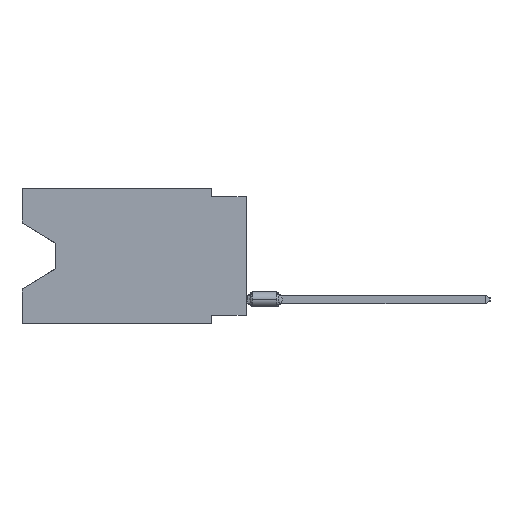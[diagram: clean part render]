
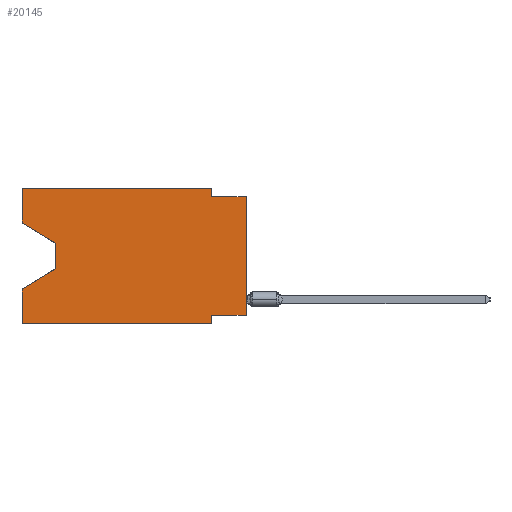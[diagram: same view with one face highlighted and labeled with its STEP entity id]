
A CAD part, left-side view. The second image highlights one B-rep face of the part: STEP entity #20145.
In plain terms, the highlighted planar face has unit normal (-1, 0, 0).
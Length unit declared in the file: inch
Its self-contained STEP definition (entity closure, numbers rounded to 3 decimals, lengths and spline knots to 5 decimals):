
#179 = VERTEX_POINT ( 'NONE', #20235 ) ;
#3113 = VERTEX_POINT ( 'NONE', #60372 ) ;
#4056 = ORIENTED_EDGE ( 'NONE', *, *, #14841, .F. ) ;
#4357 = ORIENTED_EDGE ( 'NONE', *, *, #53268, .F. ) ;
#5197 = EDGE_CURVE ( 'NONE', #50415, #5740, #31365, .T. ) ;
#5271 = ORIENTED_EDGE ( 'NONE', *, *, #59676, .F. ) ;
#5649 = CARTESIAN_POINT ( 'NONE',  ( 0., 0.1, 0. ) ) ;
#5740 = VERTEX_POINT ( 'NONE', #42033 ) ;
#7003 = ORIENTED_EDGE ( 'NONE', *, *, #23905, .T. ) ;
#7552 = CARTESIAN_POINT ( 'NONE',  ( 0., 0., -0.025 ) ) ;
#7831 = VERTEX_POINT ( 'NONE', #5649 ) ;
#9618 = ORIENTED_EDGE ( 'NONE', *, *, #47656, .F. ) ;
#11013 = CARTESIAN_POINT ( 'NONE',  ( 0., 0., -0.365 ) ) ;
#12221 = VERTEX_POINT ( 'NONE', #50980 ) ;
#13421 = DIRECTION ( 'NONE',  ( 0., 0., -1. ) ) ;
#14158 = EDGE_CURVE ( 'NONE', #179, #12221, #44955, .T. ) ;
#14216 = LINE ( 'NONE', #23410, #37818 ) ;
#14841 = EDGE_CURVE ( 'NONE', #179, #50085, #43322, .T. ) ;
#14908 = VECTOR ( 'NONE', #20843, 39.37008 ) ;
#15669 = CARTESIAN_POINT ( 'NONE',  ( 0., 0., -0.025 ) ) ;
#15686 = CARTESIAN_POINT ( 'NONE',  ( 0., 0.1, -0.025 ) ) ;
#15963 = VERTEX_POINT ( 'NONE', #64631 ) ;
#17305 = VECTOR ( 'NONE', #48688, 39.37008 ) ;
#18041 = AXIS2_PLACEMENT_3D ( 'NONE', #37891, #27103, #28382 ) ;
#18329 = LINE ( 'NONE', #38347, #19926 ) ;
#18697 = CARTESIAN_POINT ( 'NONE',  ( 0., 0.645, 0. ) ) ;
#19677 = DIRECTION ( 'NONE',  ( 0., -1., 0. ) ) ;
#19894 = CARTESIAN_POINT ( 'NONE',  ( 0., 0., -0.365 ) ) ;
#19926 = VECTOR ( 'NONE', #13421, 39.37008 ) ;
#20145 = ADVANCED_FACE ( 'NONE', ( #22159 ), #32978, .F. ) ;
#20235 = CARTESIAN_POINT ( 'NONE',  ( 0., 0.645, -0.39 ) ) ;
#20764 = EDGE_CURVE ( 'NONE', #15963, #3113, #51797, .T. ) ;
#20843 = DIRECTION ( 'NONE',  ( 0., 1., 0. ) ) ;
#21814 = LINE ( 'NONE', #41856, #46612 ) ;
#22159 = FACE_OUTER_BOUND ( 'NONE', #59425, .T. ) ;
#22461 = DIRECTION ( 'NONE',  ( 0., 0., -1. ) ) ;
#23410 = CARTESIAN_POINT ( 'NONE',  ( 0., 0.55, -0.232 ) ) ;
#23905 = EDGE_CURVE ( 'NONE', #47627, #50085, #14216, .T. ) ;
#24594 = DIRECTION ( 'NONE',  ( 0., 0., 1. ) ) ;
#24716 = LINE ( 'NONE', #25043, #17305 ) ;
#25043 = CARTESIAN_POINT ( 'NONE',  ( 0., 0.55, -0.158 ) ) ;
#25071 = ORIENTED_EDGE ( 'NONE', *, *, #38906, .F. ) ;
#25339 = EDGE_CURVE ( 'NONE', #15963, #28167, #46119, .T. ) ;
#26994 = CARTESIAN_POINT ( 'NONE',  ( 0., 0.645, 0. ) ) ;
#27103 = DIRECTION ( 'NONE',  ( 1., 0., 0. ) ) ;
#27192 = CARTESIAN_POINT ( 'NONE',  ( 0., 0.645, 0. ) ) ;
#28167 = VERTEX_POINT ( 'NONE', #45970 ) ;
#28382 = DIRECTION ( 'NONE',  ( 0., 0., -1. ) ) ;
#28997 = DIRECTION ( 'NONE',  ( 0., 0.855, -0.519 ) ) ;
#29399 = ORIENTED_EDGE ( 'NONE', *, *, #5197, .F. ) ;
#31365 = LINE ( 'NONE', #11013, #14908 ) ;
#32113 = DIRECTION ( 'NONE',  ( 0., 0., 1. ) ) ;
#32447 = CARTESIAN_POINT ( 'NONE',  ( 0., 0.645, -0.28975 ) ) ;
#32720 = VECTOR ( 'NONE', #47095, 39.37008 ) ;
#32978 = PLANE ( 'NONE',  #18041 ) ;
#35094 = VERTEX_POINT ( 'NONE', #15669 ) ;
#35538 = VECTOR ( 'NONE', #19677, 39.37008 ) ;
#36519 = LINE ( 'NONE', #26994, #55409 ) ;
#37818 = VECTOR ( 'NONE', #28997, 39.37008 ) ;
#37891 = CARTESIAN_POINT ( 'NONE',  ( 0., 0.645, 0. ) ) ;
#38124 = EDGE_CURVE ( 'NONE', #28167, #47627, #24716, .T. ) ;
#38347 = CARTESIAN_POINT ( 'NONE',  ( 0., 0.1, 0. ) ) ;
#38906 = EDGE_CURVE ( 'NONE', #47852, #35094, #47889, .T. ) ;
#39566 = ORIENTED_EDGE ( 'NONE', *, *, #38124, .T. ) ;
#41256 = ORIENTED_EDGE ( 'NONE', *, *, #25339, .T. ) ;
#41856 = CARTESIAN_POINT ( 'NONE',  ( 0., 0.1, -0.39 ) ) ;
#41909 = ORIENTED_EDGE ( 'NONE', *, *, #59206, .T. ) ;
#41927 = CARTESIAN_POINT ( 'NONE',  ( 0., 0., 0. ) ) ;
#42033 = CARTESIAN_POINT ( 'NONE',  ( 0., 0.1, -0.365 ) ) ;
#43322 = LINE ( 'NONE', #18697, #60743 ) ;
#43792 = VECTOR ( 'NONE', #56022, 39.37008 ) ;
#44955 = LINE ( 'NONE', #55104, #35538 ) ;
#45970 = CARTESIAN_POINT ( 'NONE',  ( 0., 0.55, -0.158 ) ) ;
#46119 = LINE ( 'NONE', #46759, #32720 ) ;
#46612 = VECTOR ( 'NONE', #22461, 39.37008 ) ;
#46759 = CARTESIAN_POINT ( 'NONE',  ( 0., 0.645, -0.10025 ) ) ;
#47095 = DIRECTION ( 'NONE',  ( 0., -0.855, -0.519 ) ) ;
#47627 = VERTEX_POINT ( 'NONE', #58385 ) ;
#47656 = EDGE_CURVE ( 'NONE', #7831, #47852, #18329, .T. ) ;
#47852 = VERTEX_POINT ( 'NONE', #15686 ) ;
#47889 = LINE ( 'NONE', #7552, #54057 ) ;
#48688 = DIRECTION ( 'NONE',  ( 0., 0., -1. ) ) ;
#50085 = VERTEX_POINT ( 'NONE', #32447 ) ;
#50415 = VERTEX_POINT ( 'NONE', #19894 ) ;
#50980 = CARTESIAN_POINT ( 'NONE',  ( 0., 0.1, -0.39 ) ) ;
#51797 = LINE ( 'NONE', #27192, #55967 ) ;
#53268 = EDGE_CURVE ( 'NONE', #5740, #12221, #21814, .T. ) ;
#54057 = VECTOR ( 'NONE', #61699, 39.37008 ) ;
#54949 = ORIENTED_EDGE ( 'NONE', *, *, #14158, .T. ) ;
#55104 = CARTESIAN_POINT ( 'NONE',  ( 0., 0.645, -0.39 ) ) ;
#55409 = VECTOR ( 'NONE', #57174, 39.37008 ) ;
#55967 = VECTOR ( 'NONE', #32113, 39.37008 ) ;
#56022 = DIRECTION ( 'NONE',  ( 0., 0., 1. ) ) ;
#57174 = DIRECTION ( 'NONE',  ( 0., -1., 0. ) ) ;
#58385 = CARTESIAN_POINT ( 'NONE',  ( 0., 0.55, -0.232 ) ) ;
#59206 = EDGE_CURVE ( 'NONE', #50415, #35094, #61925, .T. ) ;
#59425 = EDGE_LOOP ( 'NONE', ( #41256, #39566, #7003, #4056, #54949, #4357, #29399, #41909, #25071, #9618, #5271, #60985 ) ) ;
#59676 = EDGE_CURVE ( 'NONE', #3113, #7831, #36519, .T. ) ;
#60372 = CARTESIAN_POINT ( 'NONE',  ( 0., 0.645, 0. ) ) ;
#60743 = VECTOR ( 'NONE', #24594, 39.37008 ) ;
#60985 = ORIENTED_EDGE ( 'NONE', *, *, #20764, .F. ) ;
#61699 = DIRECTION ( 'NONE',  ( 0., -1., 0. ) ) ;
#61925 = LINE ( 'NONE', #41927, #43792 ) ;
#64631 = CARTESIAN_POINT ( 'NONE',  ( 0., 0.645, -0.10025 ) ) ;
